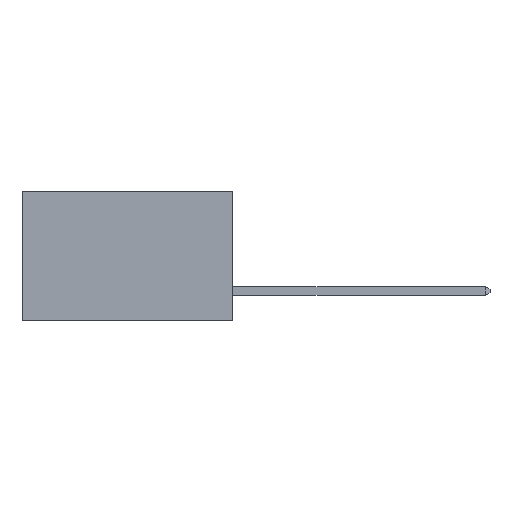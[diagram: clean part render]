
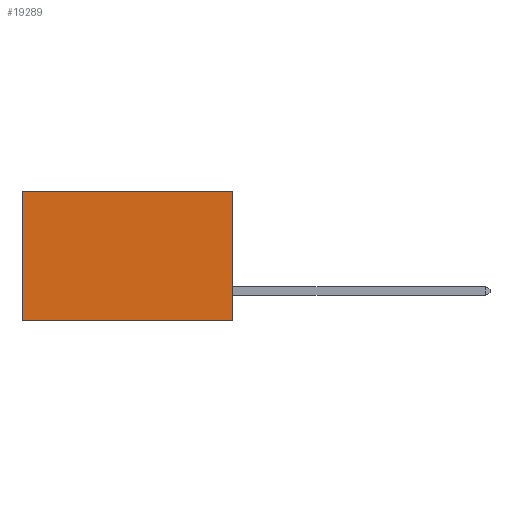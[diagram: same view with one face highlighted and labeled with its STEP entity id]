
A CAD part, left-side view. The second image highlights one B-rep face of the part: STEP entity #19289.
In plain terms, the highlighted planar face has unit normal (-1, 0, 0).
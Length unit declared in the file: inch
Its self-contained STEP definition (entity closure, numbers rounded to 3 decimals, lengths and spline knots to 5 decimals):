
#922 = VERTEX_POINT ( 'NONE', #1205 ) ;
#1205 = CARTESIAN_POINT ( 'NONE',  ( 0.2875, 0.6, 0. ) ) ;
#1643 = CARTESIAN_POINT ( 'NONE',  ( 0.2875, 0., 0. ) ) ;
#3015 = ORIENTED_EDGE ( 'NONE', *, *, #16304, .T. ) ;
#3161 = LINE ( 'NONE', #20509, #7049 ) ;
#3664 = CARTESIAN_POINT ( 'NONE',  ( 0.2875, 0., -0.37 ) ) ;
#3742 = CARTESIAN_POINT ( 'NONE',  ( 0.2875, 0.6, -0.37 ) ) ;
#4005 = DIRECTION ( 'NONE',  ( 1., 0., 0. ) ) ;
#4341 = AXIS2_PLACEMENT_3D ( 'NONE', #13717, #4005, #15298 ) ;
#5270 = DIRECTION ( 'NONE',  ( 0., 1., 0. ) ) ;
#5343 = LINE ( 'NONE', #6481, #13977 ) ;
#5576 = PLANE ( 'NONE',  #4341 ) ;
#6151 = CARTESIAN_POINT ( 'NONE',  ( 0.2875, 0.6, 0. ) ) ;
#6323 = DIRECTION ( 'NONE',  ( 0., 1., 0. ) ) ;
#6481 = CARTESIAN_POINT ( 'NONE',  ( 0.2875, 0., 0. ) ) ;
#6707 = VECTOR ( 'NONE', #14233, 39.37008 ) ;
#7049 = VECTOR ( 'NONE', #6323, 39.37008 ) ;
#7413 = ORIENTED_EDGE ( 'NONE', *, *, #17106, .F. ) ;
#7928 = CARTESIAN_POINT ( 'NONE',  ( 0.2875, 0., -0.37 ) ) ;
#9362 = VECTOR ( 'NONE', #5270, 39.37008 ) ;
#9834 = EDGE_CURVE ( 'NONE', #19048, #20598, #5343, .T. ) ;
#10930 = ORIENTED_EDGE ( 'NONE', *, *, #17829, .T. ) ;
#11234 = VERTEX_POINT ( 'NONE', #3742 ) ;
#12903 = DIRECTION ( 'NONE',  ( 0., 0., -1. ) ) ;
#13564 = ORIENTED_EDGE ( 'NONE', *, *, #9834, .F. ) ;
#13717 = CARTESIAN_POINT ( 'NONE',  ( 0.2875, 0., 0. ) ) ;
#13977 = VECTOR ( 'NONE', #12903, 39.37008 ) ;
#14233 = DIRECTION ( 'NONE',  ( 0., 0., -1. ) ) ;
#15192 = FACE_OUTER_BOUND ( 'NONE', #17839, .T. ) ;
#15298 = DIRECTION ( 'NONE',  ( 0., 0., -1. ) ) ;
#16304 = EDGE_CURVE ( 'NONE', #922, #11234, #19793, .T. ) ;
#17106 = EDGE_CURVE ( 'NONE', #20598, #11234, #17717, .T. ) ;
#17717 = LINE ( 'NONE', #3664, #9362 ) ;
#17829 = EDGE_CURVE ( 'NONE', #19048, #922, #3161, .T. ) ;
#17839 = EDGE_LOOP ( 'NONE', ( #3015, #7413, #13564, #10930 ) ) ;
#19048 = VERTEX_POINT ( 'NONE', #1643 ) ;
#19289 = ADVANCED_FACE ( 'NONE', ( #15192 ), #5576, .F. ) ;
#19793 = LINE ( 'NONE', #6151, #6707 ) ;
#20509 = CARTESIAN_POINT ( 'NONE',  ( 0.2875, 0., 0. ) ) ;
#20598 = VERTEX_POINT ( 'NONE', #7928 ) ;
